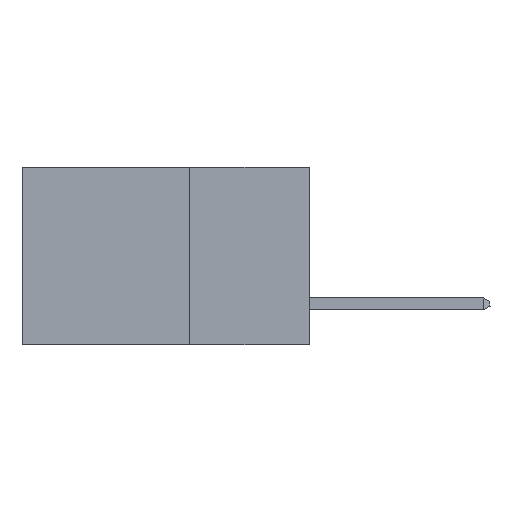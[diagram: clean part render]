
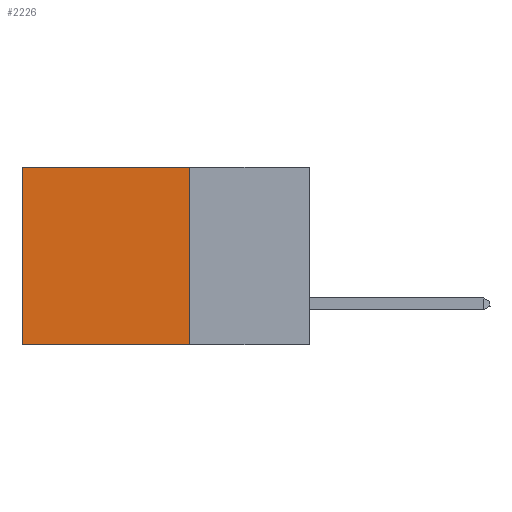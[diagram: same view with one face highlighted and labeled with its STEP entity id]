
A CAD part, left-side view. The second image highlights one B-rep face of the part: STEP entity #2226.
In plain terms, the highlighted planar face has unit normal (-1, 0, 0).
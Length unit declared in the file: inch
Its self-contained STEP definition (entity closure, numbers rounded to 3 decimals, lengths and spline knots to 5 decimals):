
#1351 = EDGE_LOOP ( 'NONE', ( #22931, #40897, #8152, #15694 ) ) ;
#2226 = ADVANCED_FACE ( 'NONE', ( #26196 ), #2524, .F. ) ;
#2524 = PLANE ( 'NONE',  #27347 ) ;
#4585 = VECTOR ( 'NONE', #29168, 39.37008 ) ;
#5327 = VERTEX_POINT ( 'NONE', #5348 ) ;
#5348 = CARTESIAN_POINT ( 'NONE',  ( 0.2875, 0.6, -0.37 ) ) ;
#7164 = DIRECTION ( 'NONE',  ( 0., 1., 0. ) ) ;
#7490 = DIRECTION ( 'NONE',  ( 1., 0., 0. ) ) ;
#8152 = ORIENTED_EDGE ( 'NONE', *, *, #11697, .F. ) ;
#10210 = CARTESIAN_POINT ( 'NONE',  ( 0.2875, 0.25, 0. ) ) ;
#10251 = CARTESIAN_POINT ( 'NONE',  ( 0.2875, 0.25, -0.37 ) ) ;
#11000 = CARTESIAN_POINT ( 'NONE',  ( 0.2875, 0.25, 0. ) ) ;
#11169 = CARTESIAN_POINT ( 'NONE',  ( 0.2875, 0.25, 0. ) ) ;
#11697 = EDGE_CURVE ( 'NONE', #13466, #44657, #29314, .T. ) ;
#13466 = VERTEX_POINT ( 'NONE', #11000 ) ;
#13613 = DIRECTION ( 'NONE',  ( 0., 0., -1. ) ) ;
#13925 = VECTOR ( 'NONE', #7164, 39.37008 ) ;
#14243 = DIRECTION ( 'NONE',  ( 0., 1., 0. ) ) ;
#14645 = EDGE_CURVE ( 'NONE', #24784, #5327, #26113, .T. ) ;
#15694 = ORIENTED_EDGE ( 'NONE', *, *, #45752, .T. ) ;
#16362 = VECTOR ( 'NONE', #13613, 39.37008 ) ;
#16458 = CARTESIAN_POINT ( 'NONE',  ( 0.2875, 0.6, 0. ) ) ;
#17957 = CARTESIAN_POINT ( 'NONE',  ( 0.2875, 0.6, 0. ) ) ;
#18259 = CARTESIAN_POINT ( 'NONE',  ( 0.2875, 0.25, 0. ) ) ;
#22931 = ORIENTED_EDGE ( 'NONE', *, *, #14645, .T. ) ;
#24784 = VERTEX_POINT ( 'NONE', #16458 ) ;
#26113 = LINE ( 'NONE', #17957, #16362 ) ;
#26196 = FACE_OUTER_BOUND ( 'NONE', #1351, .T. ) ;
#27336 = EDGE_CURVE ( 'NONE', #44657, #5327, #31725, .T. ) ;
#27347 = AXIS2_PLACEMENT_3D ( 'NONE', #18259, #7490, #44321 ) ;
#29168 = DIRECTION ( 'NONE',  ( 0., 0., -1. ) ) ;
#29314 = LINE ( 'NONE', #11169, #4585 ) ;
#29449 = LINE ( 'NONE', #10210, #13925 ) ;
#31725 = LINE ( 'NONE', #10251, #41468 ) ;
#32560 = CARTESIAN_POINT ( 'NONE',  ( 0.2875, 0.25, -0.37 ) ) ;
#40897 = ORIENTED_EDGE ( 'NONE', *, *, #27336, .F. ) ;
#41468 = VECTOR ( 'NONE', #14243, 39.37008 ) ;
#44321 = DIRECTION ( 'NONE',  ( 0., 0., -1. ) ) ;
#44657 = VERTEX_POINT ( 'NONE', #32560 ) ;
#45752 = EDGE_CURVE ( 'NONE', #13466, #24784, #29449, .T. ) ;
